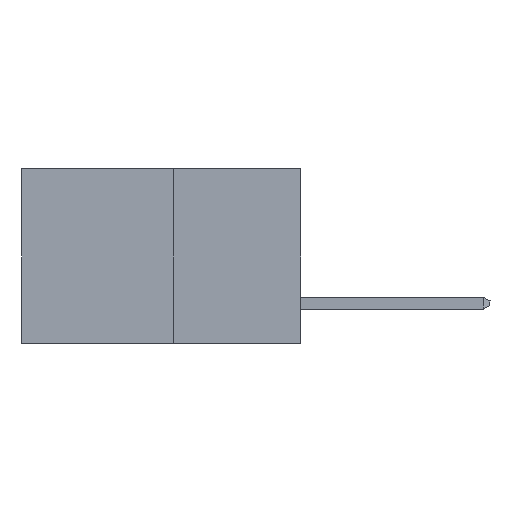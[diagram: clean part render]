
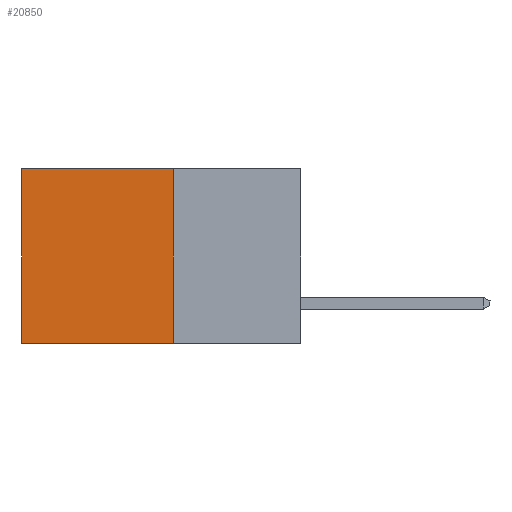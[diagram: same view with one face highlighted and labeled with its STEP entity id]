
A CAD part, left-side view. The second image highlights one B-rep face of the part: STEP entity #20850.
In plain terms, the highlighted planar face has unit normal (-1, 0, 0).
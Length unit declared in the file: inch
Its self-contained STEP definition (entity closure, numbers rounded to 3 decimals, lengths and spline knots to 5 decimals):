
#129 = ORIENTED_EDGE ( 'NONE', *, *, #25173, .F. ) ;
#1188 = LINE ( 'NONE', #30475, #27143 ) ;
#2102 = FACE_OUTER_BOUND ( 'NONE', #23302, .T. ) ;
#2642 = VECTOR ( 'NONE', #6597, 39.37008 ) ;
#4921 = DIRECTION ( 'NONE',  ( 0., 0., -1. ) ) ;
#5032 = ORIENTED_EDGE ( 'NONE', *, *, #31821, .F. ) ;
#5703 = DIRECTION ( 'NONE',  ( 0., 0., -1. ) ) ;
#6597 = DIRECTION ( 'NONE',  ( 0., 1., 0. ) ) ;
#7447 = AXIS2_PLACEMENT_3D ( 'NONE', #17639, #25234, #10220 ) ;
#10220 = DIRECTION ( 'NONE',  ( 0., 0., -1. ) ) ;
#10726 = CARTESIAN_POINT ( 'NONE',  ( 0.277, 0.27, 0. ) ) ;
#13041 = VECTOR ( 'NONE', #5703, 39.37008 ) ;
#13436 = LINE ( 'NONE', #22459, #20044 ) ;
#15717 = VERTEX_POINT ( 'NONE', #10726 ) ;
#16320 = CARTESIAN_POINT ( 'NONE',  ( 0.277, 0.27, -0.37 ) ) ;
#16572 = VERTEX_POINT ( 'NONE', #31555 ) ;
#17639 = CARTESIAN_POINT ( 'NONE',  ( 0.277, 0.27, -0.37 ) ) ;
#18179 = CARTESIAN_POINT ( 'NONE',  ( 0.277, 0.59, -0.37 ) ) ;
#19102 = VERTEX_POINT ( 'NONE', #31907 ) ;
#20044 = VECTOR ( 'NONE', #4921, 39.37008 ) ;
#20850 = ADVANCED_FACE ( 'NONE', ( #2102 ), #22676, .F. ) ;
#21213 = LINE ( 'NONE', #18179, #13041 ) ;
#22459 = CARTESIAN_POINT ( 'NONE',  ( 0.277, 0.27, -0.37 ) ) ;
#22521 = ORIENTED_EDGE ( 'NONE', *, *, #29204, .T. ) ;
#22676 = PLANE ( 'NONE',  #7447 ) ;
#23302 = EDGE_LOOP ( 'NONE', ( #25944, #5032, #129, #22521 ) ) ;
#24129 = CARTESIAN_POINT ( 'NONE',  ( 0.277, 0.27, 0. ) ) ;
#25173 = EDGE_CURVE ( 'NONE', #15717, #27804, #13436, .T. ) ;
#25234 = DIRECTION ( 'NONE',  ( 1., 0., 0. ) ) ;
#25557 = DIRECTION ( 'NONE',  ( 0., 1., 0. ) ) ;
#25944 = ORIENTED_EDGE ( 'NONE', *, *, #31863, .T. ) ;
#27143 = VECTOR ( 'NONE', #25557, 39.37008 ) ;
#27770 = LINE ( 'NONE', #24129, #2642 ) ;
#27804 = VERTEX_POINT ( 'NONE', #16320 ) ;
#29204 = EDGE_CURVE ( 'NONE', #15717, #19102, #27770, .T. ) ;
#30475 = CARTESIAN_POINT ( 'NONE',  ( 0.277, 0.27, -0.37 ) ) ;
#31555 = CARTESIAN_POINT ( 'NONE',  ( 0.277, 0.59, -0.37 ) ) ;
#31821 = EDGE_CURVE ( 'NONE', #27804, #16572, #1188, .T. ) ;
#31863 = EDGE_CURVE ( 'NONE', #19102, #16572, #21213, .T. ) ;
#31907 = CARTESIAN_POINT ( 'NONE',  ( 0.277, 0.59, 0. ) ) ;
